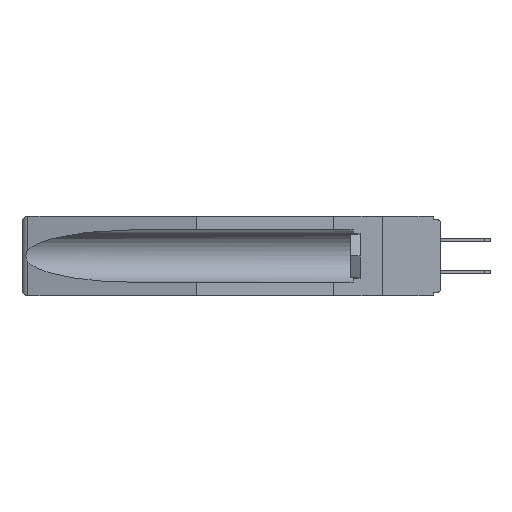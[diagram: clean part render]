
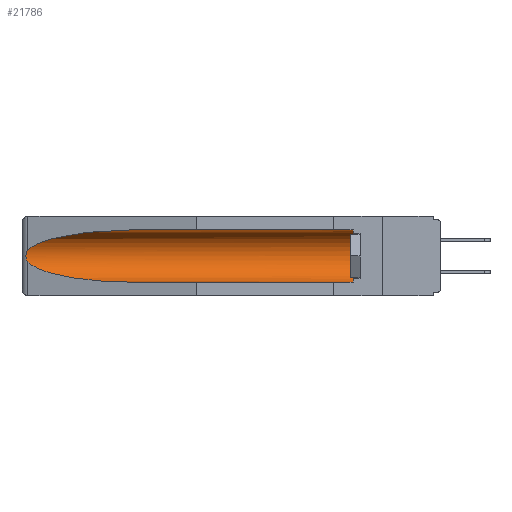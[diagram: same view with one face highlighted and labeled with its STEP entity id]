
A CAD part, left-side view. The second image highlights one B-rep face of the part: STEP entity #21786.
In plain terms, the highlighted cylindrical face has radius 2.857 mm (diameter 5.715 mm), a partial arc.
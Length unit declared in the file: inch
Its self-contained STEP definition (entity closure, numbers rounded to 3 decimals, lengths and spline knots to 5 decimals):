
#217 = VERTEX_POINT ( 'NONE', #13903 ) ;
#266 = AXIS2_PLACEMENT_3D ( 'NONE', #4948, #1089, #6849 ) ;
#481 = DIRECTION ( 'NONE',  ( 0., 1., 0. ) ) ;
#1089 = DIRECTION ( 'NONE',  ( 0., -1., 0. ) ) ;
#1353 = VECTOR ( 'NONE', #4481, 39.37008 ) ;
#1360 = CARTESIAN_POINT ( 'NONE',  ( 0.155, 0.126, -0.284 ) ) ;
#1627 =( BOUNDED_CURVE ( )  B_SPLINE_CURVE ( 3, ( #13950, #22974, #6327, #11808 ),
 .UNSPECIFIED., .F., .F. ) 
 B_SPLINE_CURVE_WITH_KNOTS ( ( 4, 4 ),
 ( 0.1948, 1.5708 ),
 .UNSPECIFIED. ) 
 CURVE ( )  GEOMETRIC_REPRESENTATION_ITEM ( )  RATIONAL_B_SPLINE_CURVE ( ( 1., 0.848, 0.848, 1. ) ) 
 REPRESENTATION_ITEM ( '' )  );
#1838 = EDGE_CURVE ( 'NONE', #13177, #217, #15848, .T. ) ;
#2252 = CARTESIAN_POINT ( 'NONE',  ( 0.155, -0.30754, -0.059 ) ) ;
#3564 = CARTESIAN_POINT ( 'NONE',  ( 0.21114, 1.30732, -0.059 ) ) ;
#3665 = LINE ( 'NONE', #11538, #1353 ) ;
#3900 = CARTESIAN_POINT ( 'NONE',  ( 0.155, 0.126, -0.059 ) ) ;
#4362 = ORIENTED_EDGE ( 'NONE', *, *, #1838, .T. ) ;
#4481 = DIRECTION ( 'NONE',  ( 0., 1., 0. ) ) ;
#4572 = EDGE_CURVE ( 'NONE', #7409, #10120, #3665, .T. ) ;
#4948 = CARTESIAN_POINT ( 'NONE',  ( 0.155, 0.126, -0.1715 ) ) ;
#5090 = EDGE_CURVE ( 'NONE', #7409, #15996, #13373, .T. ) ;
#5711 = DIRECTION ( 'NONE',  ( 0., 1., 0. ) ) ;
#6327 = CARTESIAN_POINT ( 'NONE',  ( 0.21114, 1.30732, -0.284 ) ) ;
#6410 = AXIS2_PLACEMENT_3D ( 'NONE', #7668, #481, #13297 ) ;
#6849 = DIRECTION ( 'NONE',  ( 0., 0., 1. ) ) ;
#7144 = EDGE_CURVE ( 'NONE', #217, #10120, #1627, .T. ) ;
#7409 = VERTEX_POINT ( 'NONE', #1360 ) ;
#7668 = CARTESIAN_POINT ( 'NONE',  ( 0.155, -0.30754, -0.1715 ) ) ;
#7938 = CARTESIAN_POINT ( 'NONE',  ( 0.26655, 1.53094, -0.18657 ) ) ;
#8782 = CYLINDRICAL_SURFACE ( 'NONE', #6410, 0.1125 ) ;
#10120 = VERTEX_POINT ( 'NONE', #15577 ) ;
#10616 = ORIENTED_EDGE ( 'NONE', *, *, #20556, .T. ) ;
#10630 = VECTOR ( 'NONE', #5711, 39.37008 ) ;
#11168 = CARTESIAN_POINT ( 'NONE',  ( 0.26654, 1.53092, -0.15636 ) ) ;
#11327 = CARTESIAN_POINT ( 'NONE',  ( 0.26537, 1.52718, -0.14972 ) ) ;
#11538 = CARTESIAN_POINT ( 'NONE',  ( 0.155, -0.30754, -0.284 ) ) ;
#11559 = CARTESIAN_POINT ( 'NONE',  ( 0.2675, 1.53308, -0.17534 ) ) ;
#11642 = CARTESIAN_POINT ( 'NONE',  ( 0.2675, 1.53308, -0.16763 ) ) ;
#11808 = CARTESIAN_POINT ( 'NONE',  ( 0.155, 1.07973, -0.284 ) ) ;
#12422 = EDGE_LOOP ( 'NONE', ( #10616, #4362, #19848, #16754, #21611, #15986 ) ) ;
#13177 = VERTEX_POINT ( 'NONE', #13242 ) ;
#13225 = EDGE_CURVE ( 'NONE', #15996, #14196, #23625, .T. ) ;
#13242 = CARTESIAN_POINT ( 'NONE',  ( 0.26537, 1.52718, -0.14972 ) ) ;
#13297 = DIRECTION ( 'NONE',  ( 0., 0., 1. ) ) ;
#13373 = CIRCLE ( 'NONE', #266, 0.1125 ) ;
#13903 = CARTESIAN_POINT ( 'NONE',  ( 0.26537, 1.52718, -0.19328 ) ) ;
#13950 = CARTESIAN_POINT ( 'NONE',  ( 0.26537, 1.52718, -0.19328 ) ) ;
#14196 = VERTEX_POINT ( 'NONE', #17803 ) ;
#14954 = CARTESIAN_POINT ( 'NONE',  ( 0.2673, 1.5327, -0.16383 ) ) ;
#15577 = CARTESIAN_POINT ( 'NONE',  ( 0.155, 1.07973, -0.284 ) ) ;
#15848 = B_SPLINE_CURVE_WITH_KNOTS ( 'NONE', 3,
 ( #11327, #22191, #11168, #14954, #11642, #11559, #16892, #7938, #20570, #20722 ),
 .UNSPECIFIED., .F., .F.,
 ( 4, 2, 2, 2, 4 ),
 ( 0., 0.00029, 0.00058, 0.00087, 0.00117 ),
 .UNSPECIFIED. ) ;
#15986 = ORIENTED_EDGE ( 'NONE', *, *, #13225, .T. ) ;
#15996 = VERTEX_POINT ( 'NONE', #3900 ) ;
#16754 = ORIENTED_EDGE ( 'NONE', *, *, #4572, .F. ) ;
#16892 = CARTESIAN_POINT ( 'NONE',  ( 0.2673, 1.53269, -0.17917 ) ) ;
#17803 = CARTESIAN_POINT ( 'NONE',  ( 0.155, 1.07973, -0.059 ) ) ;
#18088 = CARTESIAN_POINT ( 'NONE',  ( 0.26537, 1.52718, -0.14972 ) ) ;
#18414 = CARTESIAN_POINT ( 'NONE',  ( 0.155, 1.07973, -0.059 ) ) ;
#19166 = FACE_OUTER_BOUND ( 'NONE', #12422, .T. ) ;
#19848 = ORIENTED_EDGE ( 'NONE', *, *, #7144, .T. ) ;
#20556 = EDGE_CURVE ( 'NONE', #14196, #13177, #23695, .T. ) ;
#20570 = CARTESIAN_POINT ( 'NONE',  ( 0.26597, 1.5296, -0.19026 ) ) ;
#20722 = CARTESIAN_POINT ( 'NONE',  ( 0.26537, 1.52718, -0.19328 ) ) ;
#21611 = ORIENTED_EDGE ( 'NONE', *, *, #5090, .T. ) ;
#21786 = ADVANCED_FACE ( 'NONE', ( #19166 ), #8782, .F. ) ;
#22191 = CARTESIAN_POINT ( 'NONE',  ( 0.26597, 1.52961, -0.15275 ) ) ;
#22974 = CARTESIAN_POINT ( 'NONE',  ( 0.25451, 1.48313, -0.24835 ) ) ;
#23625 = LINE ( 'NONE', #2252, #10630 ) ;
#23695 =( BOUNDED_CURVE ( )  B_SPLINE_CURVE ( 3, ( #18414, #3564, #23720, #18088 ),
 .UNSPECIFIED., .F., .F. ) 
 B_SPLINE_CURVE_WITH_KNOTS ( ( 4, 4 ),
 ( 4.71239, 6.08839 ),
 .UNSPECIFIED. ) 
 CURVE ( )  GEOMETRIC_REPRESENTATION_ITEM ( )  RATIONAL_B_SPLINE_CURVE ( ( 1., 0.848, 0.848, 1. ) ) 
 REPRESENTATION_ITEM ( '' )  );
#23720 = CARTESIAN_POINT ( 'NONE',  ( 0.25451, 1.48313, -0.09465 ) ) ;
